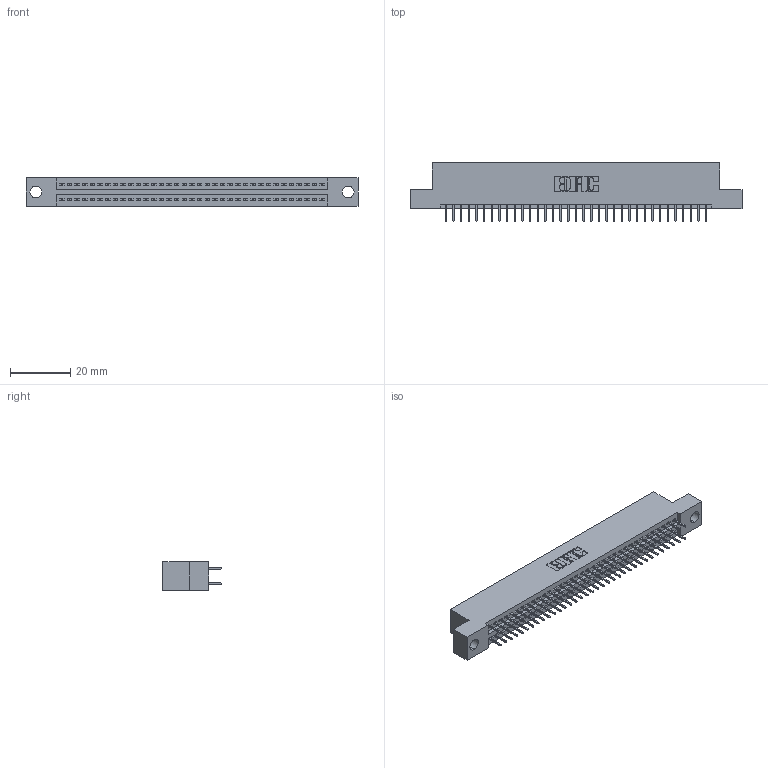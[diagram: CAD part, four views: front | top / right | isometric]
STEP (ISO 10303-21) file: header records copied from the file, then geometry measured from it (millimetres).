
FILE_DESCRIPTION (( 'STEP AP203' ), '1' );
FILE_NAME ('345-070-524-204.STEP', '2021-05-20T08:14:16', ( '' ), ( '' ), 'SwSTEP 2.0', 'SolidWorks 2020', '' );
FILE_SCHEMA (( 'CONFIG_CONTROL_DESIGN' ));
Length unit declared in the file: inch
Products named in the file (3): 345-070-524-204; 345-292-001_345-293-124; 345 Part_Flush Mounting Lugs - 0.156 Dia-TI
Assembly tree (71 placements, depth 2):
  345-070-524-204
    345 Part_Flush Mounting Lugs - 0.156 Dia-TI
    345-292-001_345-293-124  x70
Bounding box: 110.11 x 19.35 x 9.4 mm (x, y, z)
Volume: 10419.2 mm3; surface area: 14837.8 mm2
Topology: 71 solids, 71 shells, 3920 faces, 11087 edges, 7110 vertices
Faces by surface type: plane 2824, cylinder 1096
Entity records: 28897 total; most frequent: CARTESIAN_POINT 4854, ORIENTED_EDGE 4786, DIRECTION 4289, EDGE_CURVE 2393, VECTOR 2125, LINE 2125, VERTEX_POINT 1590, AXIS2_PLACEMENT_3D 1082
